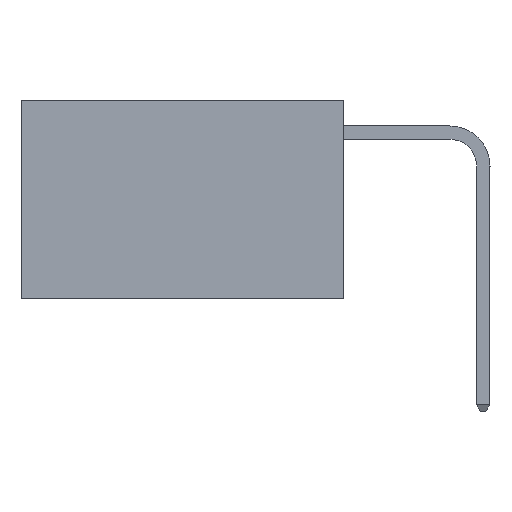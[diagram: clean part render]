
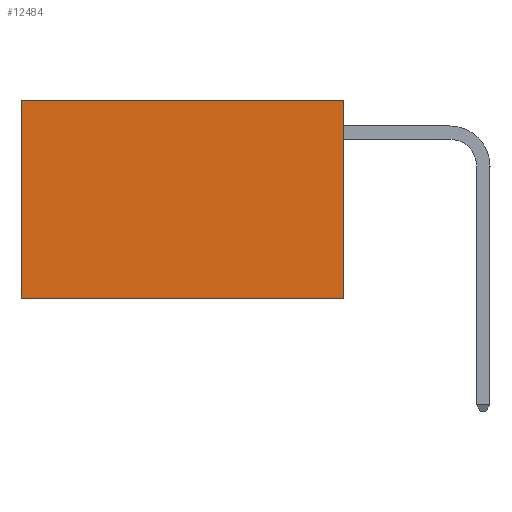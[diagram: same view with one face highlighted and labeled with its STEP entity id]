
A CAD part, left-side view. The second image highlights one B-rep face of the part: STEP entity #12484.
In plain terms, the highlighted planar face has unit normal (-1, 0, 0).
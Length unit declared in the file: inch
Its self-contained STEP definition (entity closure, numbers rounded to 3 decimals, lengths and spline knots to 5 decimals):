
#464 = DIRECTION ( 'NONE',  ( 1., 0., 0. ) ) ;
#1947 = ORIENTED_EDGE ( 'NONE', *, *, #7402, .T. ) ;
#2774 = EDGE_LOOP ( 'NONE', ( #1947, #13147, #19312, #10601 ) ) ;
#2853 = DIRECTION ( 'NONE',  ( 0., 1., 0. ) ) ;
#4619 = CARTESIAN_POINT ( 'NONE',  ( 0.2625, 0., -0.37 ) ) ;
#5171 = VECTOR ( 'NONE', #21329, 39.37008 ) ;
#6290 = LINE ( 'NONE', #14171, #5171 ) ;
#6937 = VERTEX_POINT ( 'NONE', #8999 ) ;
#6986 = DIRECTION ( 'NONE',  ( 0., 0., -1. ) ) ;
#7099 = EDGE_CURVE ( 'NONE', #6937, #10349, #15899, .T. ) ;
#7402 = EDGE_CURVE ( 'NONE', #22658, #10349, #6290, .T. ) ;
#8294 = EDGE_CURVE ( 'NONE', #17534, #22658, #13383, .T. ) ;
#8999 = CARTESIAN_POINT ( 'NONE',  ( 0.2625, 0., -0.37 ) ) ;
#10349 = VERTEX_POINT ( 'NONE', #13711 ) ;
#10522 = CARTESIAN_POINT ( 'NONE',  ( 0.2625, 0., 0. ) ) ;
#10601 = ORIENTED_EDGE ( 'NONE', *, *, #8294, .T. ) ;
#11206 = CARTESIAN_POINT ( 'NONE',  ( 0.2625, 0., 0. ) ) ;
#11832 = VECTOR ( 'NONE', #2853, 39.37008 ) ;
#12244 = EDGE_CURVE ( 'NONE', #17534, #6937, #20730, .T. ) ;
#12484 = ADVANCED_FACE ( 'NONE', ( #15192 ), #19923, .F. ) ;
#12519 = VECTOR ( 'NONE', #6986, 39.37008 ) ;
#12941 = DIRECTION ( 'NONE',  ( 0., 0., -1. ) ) ;
#13147 = ORIENTED_EDGE ( 'NONE', *, *, #7099, .F. ) ;
#13383 = LINE ( 'NONE', #20204, #22188 ) ;
#13711 = CARTESIAN_POINT ( 'NONE',  ( 0.2625, 0.6, -0.37 ) ) ;
#14171 = CARTESIAN_POINT ( 'NONE',  ( 0.2625, 0.6, 0. ) ) ;
#14817 = AXIS2_PLACEMENT_3D ( 'NONE', #11206, #464, #12941 ) ;
#15192 = FACE_OUTER_BOUND ( 'NONE', #2774, .T. ) ;
#15899 = LINE ( 'NONE', #4619, #11832 ) ;
#17534 = VERTEX_POINT ( 'NONE', #20743 ) ;
#19312 = ORIENTED_EDGE ( 'NONE', *, *, #12244, .F. ) ;
#19923 = PLANE ( 'NONE',  #14817 ) ;
#20204 = CARTESIAN_POINT ( 'NONE',  ( 0.2625, 0., 0. ) ) ;
#20730 = LINE ( 'NONE', #10522, #12519 ) ;
#20743 = CARTESIAN_POINT ( 'NONE',  ( 0.2625, 0., 0. ) ) ;
#21329 = DIRECTION ( 'NONE',  ( 0., 0., -1. ) ) ;
#21983 = DIRECTION ( 'NONE',  ( 0., 1., 0. ) ) ;
#22188 = VECTOR ( 'NONE', #21983, 39.37008 ) ;
#22658 = VERTEX_POINT ( 'NONE', #22939 ) ;
#22939 = CARTESIAN_POINT ( 'NONE',  ( 0.2625, 0.6, 0. ) ) ;
